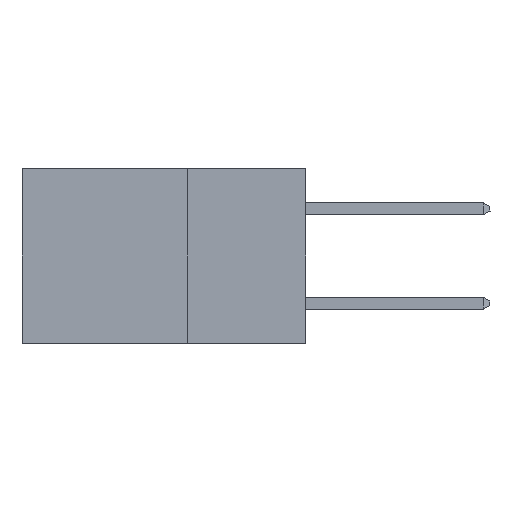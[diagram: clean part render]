
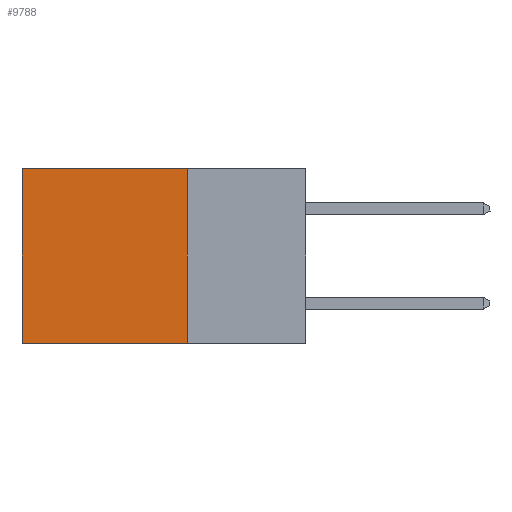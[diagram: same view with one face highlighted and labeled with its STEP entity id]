
A CAD part, left-side view. The second image highlights one B-rep face of the part: STEP entity #9788.
In plain terms, the highlighted planar face has unit normal (-1, 0, 0).
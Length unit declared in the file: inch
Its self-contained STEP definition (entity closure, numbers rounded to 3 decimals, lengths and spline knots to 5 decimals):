
#939 = LINE ( 'NONE', #5844, #14126 ) ;
#1410 = ORIENTED_EDGE ( 'NONE', *, *, #13018, .F. ) ;
#1584 = LINE ( 'NONE', #12349, #4703 ) ;
#1929 = DIRECTION ( 'NONE',  ( 0., 0., -1. ) ) ;
#3210 = VERTEX_POINT ( 'NONE', #12889 ) ;
#3475 = CARTESIAN_POINT ( 'NONE',  ( 0.298, 0.25, 0. ) ) ;
#4036 = VERTEX_POINT ( 'NONE', #13552 ) ;
#4654 = VERTEX_POINT ( 'NONE', #11249 ) ;
#4695 = EDGE_LOOP ( 'NONE', ( #13627, #1410, #16867, #16507 ) ) ;
#4703 = VECTOR ( 'NONE', #1929, 39.37008 ) ;
#5531 = EDGE_CURVE ( 'NONE', #4654, #3210, #16325, .T. ) ;
#5844 = CARTESIAN_POINT ( 'NONE',  ( 0.298, 0.6, 0. ) ) ;
#7256 = CARTESIAN_POINT ( 'NONE',  ( 0.298, 0.25, -0.37 ) ) ;
#7342 = PLANE ( 'NONE',  #8909 ) ;
#8909 = AXIS2_PLACEMENT_3D ( 'NONE', #3475, #13932, #16638 ) ;
#9102 = EDGE_CURVE ( 'NONE', #4654, #4036, #1584, .T. ) ;
#9564 = VECTOR ( 'NONE', #9726, 39.37008 ) ;
#9709 = EDGE_CURVE ( 'NONE', #3210, #10765, #939, .T. ) ;
#9726 = DIRECTION ( 'NONE',  ( 0., 1., 0. ) ) ;
#9788 = ADVANCED_FACE ( 'NONE', ( #10603 ), #7342, .F. ) ;
#10162 = VECTOR ( 'NONE', #10483, 39.37008 ) ;
#10483 = DIRECTION ( 'NONE',  ( 0., 1., 0. ) ) ;
#10603 = FACE_OUTER_BOUND ( 'NONE', #4695, .T. ) ;
#10765 = VERTEX_POINT ( 'NONE', #15135 ) ;
#11249 = CARTESIAN_POINT ( 'NONE',  ( 0.298, 0.25, 0. ) ) ;
#11874 = CARTESIAN_POINT ( 'NONE',  ( 0.298, 0.25, 0. ) ) ;
#12212 = DIRECTION ( 'NONE',  ( 0., 0., -1. ) ) ;
#12349 = CARTESIAN_POINT ( 'NONE',  ( 0.298, 0.25, 0. ) ) ;
#12646 = LINE ( 'NONE', #7256, #9564 ) ;
#12889 = CARTESIAN_POINT ( 'NONE',  ( 0.298, 0.6, 0. ) ) ;
#13018 = EDGE_CURVE ( 'NONE', #4036, #10765, #12646, .T. ) ;
#13552 = CARTESIAN_POINT ( 'NONE',  ( 0.298, 0.25, -0.37 ) ) ;
#13627 = ORIENTED_EDGE ( 'NONE', *, *, #9709, .T. ) ;
#13932 = DIRECTION ( 'NONE',  ( 1., 0., 0. ) ) ;
#14126 = VECTOR ( 'NONE', #12212, 39.37008 ) ;
#15135 = CARTESIAN_POINT ( 'NONE',  ( 0.298, 0.6, -0.37 ) ) ;
#16325 = LINE ( 'NONE', #11874, #10162 ) ;
#16507 = ORIENTED_EDGE ( 'NONE', *, *, #5531, .T. ) ;
#16638 = DIRECTION ( 'NONE',  ( 0., 0., -1. ) ) ;
#16867 = ORIENTED_EDGE ( 'NONE', *, *, #9102, .F. ) ;
